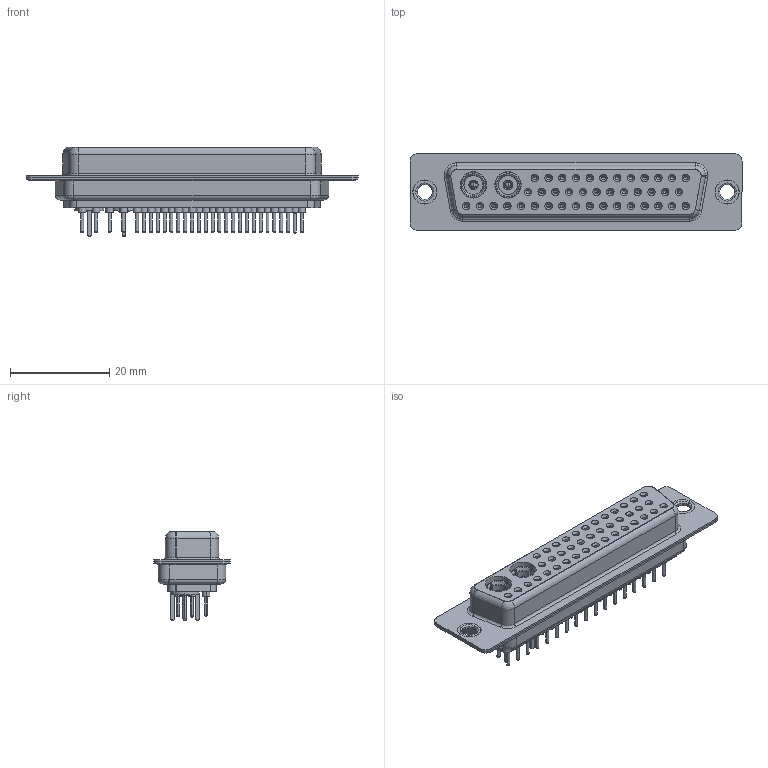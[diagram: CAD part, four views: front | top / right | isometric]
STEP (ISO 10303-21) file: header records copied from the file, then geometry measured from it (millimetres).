
FILE_DESCRIPTION (( 'STEP AP203' ), '1' );
FILE_NAME ('628-43W2624-5N1.STEP', '2019-06-26T21:15:12', ( '' ), ( '' ), 'SwSTEP 2.0', 'SolidWorks 2016', '' );
FILE_SCHEMA (( 'CONFIG_CONTROL_DESIGN' ));
Length unit declared in the file: millimetre
Products named in the file (13): 628Combo Contact Row 3_24; 628Combo Thru Hole Rivet; Co-Ax Plug Assy_St; Co-Ax Plug_Straight PC Tail; 628Combo Contact Row 1_24; 628-43W2624-5N1; Locking Collar; 628Combo Housing_43W2; 628Combo Shell Rear_50 Contacts; 628Combo Shell Front_50 Contacts; Pin_Str; Insulator Pin_Straight PC Tail; 628Combo Contact Row 2_24
Assembly tree (52 placements, depth 3):
  628-43W2624-5N1
    628Combo Housing_43W2
    628Combo Shell Front_50 Contacts
    628Combo Shell Rear_50 Contacts
    628Combo Thru Hole Rivet  x2
    628Combo Contact Row 1_24  x12
    628Combo Contact Row 2_24  x12
    628Combo Contact Row 3_24  x17
    Co-Ax Plug Assy_St  x2
      Co-Ax Plug_Straight PC Tail
      Insulator Pin_Straight PC Tail
      Pin_Str
      Locking Collar
Bounding box: 67 x 15.4 x 18.15 mm (x, y, z)
Volume: 6852.1 mm3; surface area: 14835.8 mm2
Topology: 54 solids, 54 shells, 2762 faces, 6379 edges, 3916 vertices
Faces by surface type: cylinder 990, plane 796, torus 647, cone 317, sphere 8, bspline 4
Entity records: 32090 total; most frequent: DIRECTION 5722, CARTESIAN_POINT 5248, ORIENTED_EDGE 4620, AXIS2_PLACEMENT_3D 2423, EDGE_CURVE 2310, VERTEX_POINT 1464, CIRCLE 1345, EDGE_LOOP 1284
